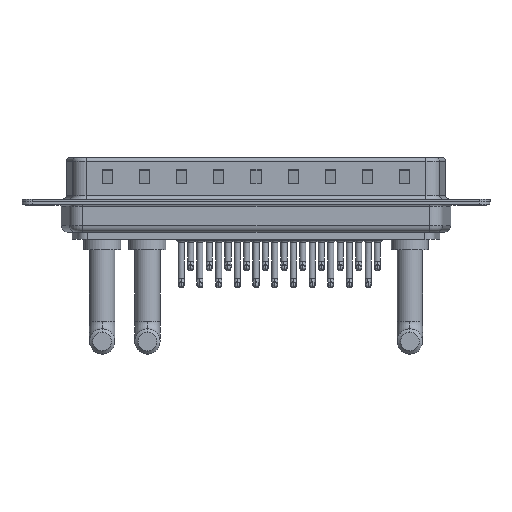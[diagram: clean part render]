
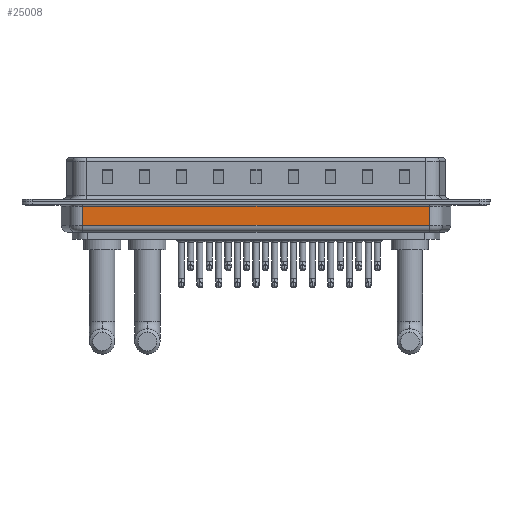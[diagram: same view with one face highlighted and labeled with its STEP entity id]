
A CAD part, front view. The second image highlights one B-rep face of the part: STEP entity #25008.
In plain terms, the highlighted planar face has unit normal (0, -1, 0).
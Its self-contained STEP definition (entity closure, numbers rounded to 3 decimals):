
#294 = LINE ( 'NONE', #22478, #8222 ) ;
#333 = LINE ( 'NONE', #12089, #1010 ) ;
#919 = DIRECTION ( 'NONE',  ( 0., 1., 0. ) ) ;
#1010 = VECTOR ( 'NONE', #7988, 1000. ) ;
#3027 = CARTESIAN_POINT ( 'NONE',  ( 6.031, -5.35, -3.5 ) ) ;
#3885 = VECTOR ( 'NONE', #17920, 1000. ) ;
#3886 = CARTESIAN_POINT ( 'NONE',  ( 57.469, -5.35, -3.5 ) ) ;
#4880 = CARTESIAN_POINT ( 'NONE',  ( 6.031, -5.35, -4.5 ) ) ;
#5268 = PLANE ( 'NONE',  #7382 ) ;
#6285 = VERTEX_POINT ( 'NONE', #8525 ) ;
#7009 = LINE ( 'NONE', #3027, #12442 ) ;
#7382 = AXIS2_PLACEMENT_3D ( 'NONE', #4880, #919, #19281 ) ;
#7988 = DIRECTION ( 'NONE',  ( 0., 0., 1. ) ) ;
#8222 = VECTOR ( 'NONE', #22343, 1000. ) ;
#8405 = ORIENTED_EDGE ( 'NONE', *, *, #17216, .T. ) ;
#8525 = CARTESIAN_POINT ( 'NONE',  ( 57.469, -5.35, -0.65 ) ) ;
#9640 = ORIENTED_EDGE ( 'NONE', *, *, #14981, .F. ) ;
#10950 = ORIENTED_EDGE ( 'NONE', *, *, #12088, .T. ) ;
#11280 = CARTESIAN_POINT ( 'NONE',  ( 6.031, -5.35, -0.65 ) ) ;
#12088 = EDGE_CURVE ( 'NONE', #18948, #6285, #17778, .T. ) ;
#12089 = CARTESIAN_POINT ( 'NONE',  ( 6.031, -5.35, -4.5 ) ) ;
#12442 = VECTOR ( 'NONE', #17025, 1000. ) ;
#14981 = EDGE_CURVE ( 'NONE', #21922, #24671, #333, .T. ) ;
#17025 = DIRECTION ( 'NONE',  ( 1., 0., 0. ) ) ;
#17216 = EDGE_CURVE ( 'NONE', #6285, #24671, #294, .T. ) ;
#17778 = LINE ( 'NONE', #25860, #3885 ) ;
#17920 = DIRECTION ( 'NONE',  ( 0., 0., 1. ) ) ;
#18948 = VERTEX_POINT ( 'NONE', #3886 ) ;
#19281 = DIRECTION ( 'NONE',  ( -1., 0., 0. ) ) ;
#20138 = ORIENTED_EDGE ( 'NONE', *, *, #25005, .T. ) ;
#21922 = VERTEX_POINT ( 'NONE', #22464 ) ;
#22343 = DIRECTION ( 'NONE',  ( -1., 0., 0. ) ) ;
#22464 = CARTESIAN_POINT ( 'NONE',  ( 6.031, -5.35, -3.5 ) ) ;
#22478 = CARTESIAN_POINT ( 'NONE',  ( 6.031, -5.35, -0.65 ) ) ;
#22995 = FACE_OUTER_BOUND ( 'NONE', #25785, .T. ) ;
#24671 = VERTEX_POINT ( 'NONE', #11280 ) ;
#25005 = EDGE_CURVE ( 'NONE', #21922, #18948, #7009, .T. ) ;
#25008 = ADVANCED_FACE ( 'NONE', ( #22995 ), #5268, .F. ) ;
#25785 = EDGE_LOOP ( 'NONE', ( #9640, #20138, #10950, #8405 ) ) ;
#25860 = CARTESIAN_POINT ( 'NONE',  ( 57.469, -5.35, -4.5 ) ) ;
